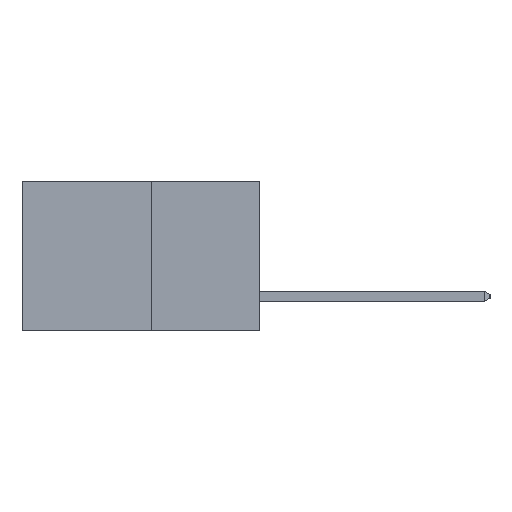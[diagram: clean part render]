
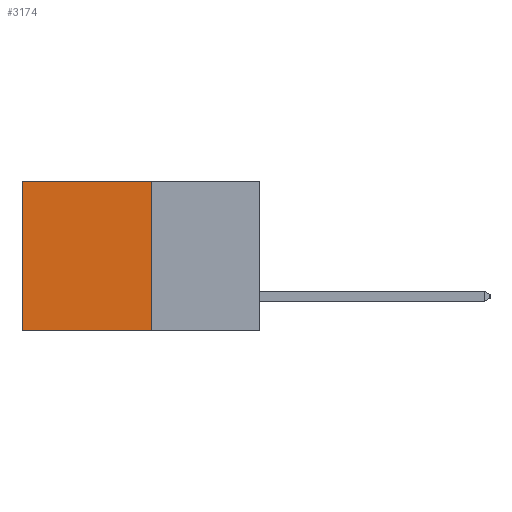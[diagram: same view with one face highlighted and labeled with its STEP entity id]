
A CAD part, left-side view. The second image highlights one B-rep face of the part: STEP entity #3174.
In plain terms, the highlighted planar face has unit normal (-1, 0, 0).
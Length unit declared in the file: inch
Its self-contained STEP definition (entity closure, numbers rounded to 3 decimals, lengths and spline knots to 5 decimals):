
#2162 = DIRECTION ( 'NONE',  ( 0., 1., 0. ) ) ;
#2453 = DIRECTION ( 'NONE',  ( 0., 0., -1. ) ) ;
#2633 = LINE ( 'NONE', #17282, #12191 ) ;
#2922 = FACE_OUTER_BOUND ( 'NONE', #16112, .T. ) ;
#3174 = ADVANCED_FACE ( 'NONE', ( #2922 ), #20665, .F. ) ;
#3991 = AXIS2_PLACEMENT_3D ( 'NONE', #20619, #20596, #20546 ) ;
#4006 = EDGE_CURVE ( 'NONE', #11333, #12274, #17601, .T. ) ;
#4476 = DIRECTION ( 'NONE',  ( 0., 0., -1. ) ) ;
#4502 = CARTESIAN_POINT ( 'NONE',  ( 0.277, 0.27, -0.37 ) ) ;
#4524 = CARTESIAN_POINT ( 'NONE',  ( 0.277, 0.27, -0.37 ) ) ;
#6418 = ORIENTED_EDGE ( 'NONE', *, *, #18767, .T. ) ;
#6516 = CARTESIAN_POINT ( 'NONE',  ( 0.277, 0.59, 0. ) ) ;
#6715 = DIRECTION ( 'NONE',  ( 0., 1., 0. ) ) ;
#7243 = CARTESIAN_POINT ( 'NONE',  ( 0.277, 0.59, -0.37 ) ) ;
#7344 = LINE ( 'NONE', #13195, #16163 ) ;
#7569 = EDGE_CURVE ( 'NONE', #12274, #18021, #2633, .T. ) ;
#8892 = CARTESIAN_POINT ( 'NONE',  ( 0.277, 0.27, 0. ) ) ;
#11333 = VERTEX_POINT ( 'NONE', #8892 ) ;
#12191 = VECTOR ( 'NONE', #6715, 39.37008 ) ;
#12252 = ORIENTED_EDGE ( 'NONE', *, *, #4006, .F. ) ;
#12274 = VERTEX_POINT ( 'NONE', #4524 ) ;
#12706 = ORIENTED_EDGE ( 'NONE', *, *, #7569, .F. ) ;
#13195 = CARTESIAN_POINT ( 'NONE',  ( 0.277, 0.59, -0.37 ) ) ;
#13528 = VECTOR ( 'NONE', #4476, 39.37008 ) ;
#14545 = LINE ( 'NONE', #19825, #18062 ) ;
#14784 = VERTEX_POINT ( 'NONE', #6516 ) ;
#16112 = EDGE_LOOP ( 'NONE', ( #19838, #12706, #12252, #6418 ) ) ;
#16163 = VECTOR ( 'NONE', #2453, 39.37008 ) ;
#17282 = CARTESIAN_POINT ( 'NONE',  ( 0.277, 0.27, -0.37 ) ) ;
#17593 = EDGE_CURVE ( 'NONE', #14784, #18021, #7344, .T. ) ;
#17601 = LINE ( 'NONE', #4502, #13528 ) ;
#18021 = VERTEX_POINT ( 'NONE', #7243 ) ;
#18062 = VECTOR ( 'NONE', #2162, 39.37008 ) ;
#18767 = EDGE_CURVE ( 'NONE', #11333, #14784, #14545, .T. ) ;
#19825 = CARTESIAN_POINT ( 'NONE',  ( 0.277, 0.27, 0. ) ) ;
#19838 = ORIENTED_EDGE ( 'NONE', *, *, #17593, .T. ) ;
#20546 = DIRECTION ( 'NONE',  ( 0., 0., -1. ) ) ;
#20596 = DIRECTION ( 'NONE',  ( 1., 0., 0. ) ) ;
#20619 = CARTESIAN_POINT ( 'NONE',  ( 0.277, 0.27, -0.37 ) ) ;
#20665 = PLANE ( 'NONE',  #3991 ) ;
